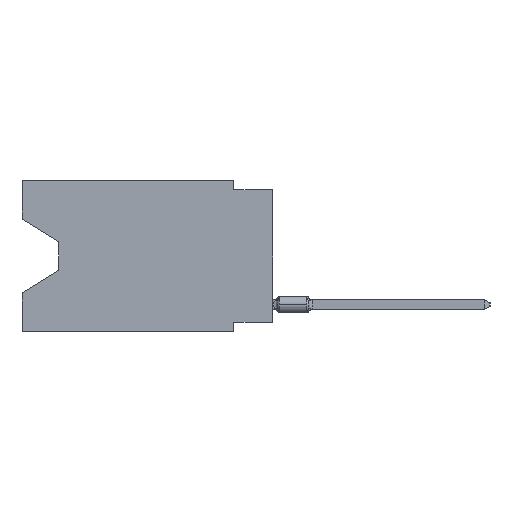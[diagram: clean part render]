
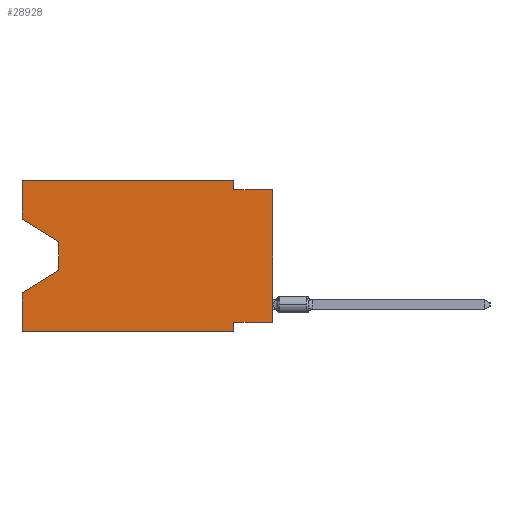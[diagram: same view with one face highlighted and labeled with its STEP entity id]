
A CAD part, left-side view. The second image highlights one B-rep face of the part: STEP entity #28928.
In plain terms, the highlighted planar face has unit normal (-1, 0, 0).
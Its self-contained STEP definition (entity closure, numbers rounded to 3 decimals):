
#574 = CARTESIAN_POINT ( 'NONE',  ( 0., 13.97, -4.013 ) ) ;
#907 = CARTESIAN_POINT ( 'NONE',  ( 0., 16.383, -7.36 ) ) ;
#1295 = DIRECTION ( 'NONE',  ( 0., -0.855, -0.519 ) ) ;
#1800 = VECTOR ( 'NONE', #1828, 1000. ) ;
#1828 = DIRECTION ( 'NONE',  ( 0., 1., 0. ) ) ;
#1912 = VECTOR ( 'NONE', #26800, 1000. ) ;
#1988 = AXIS2_PLACEMENT_3D ( 'NONE', #5019, #26627, #13633 ) ;
#2088 = EDGE_CURVE ( 'NONE', #6291, #32287, #13755, .T. ) ;
#2359 = CARTESIAN_POINT ( 'NONE',  ( 0., 16.383, -9.906 ) ) ;
#2468 = EDGE_CURVE ( 'NONE', #8703, #30453, #21940, .T. ) ;
#2623 = LINE ( 'NONE', #15472, #23914 ) ;
#2914 = CARTESIAN_POINT ( 'NONE',  ( 0., 16.383, -2.546 ) ) ;
#3420 = CARTESIAN_POINT ( 'NONE',  ( 0., 2.54, 0. ) ) ;
#3566 = ORIENTED_EDGE ( 'NONE', *, *, #20096, .T. ) ;
#3781 = DIRECTION ( 'NONE',  ( 0., 0.855, -0.519 ) ) ;
#3943 = CARTESIAN_POINT ( 'NONE',  ( 0., 2.54, -9.906 ) ) ;
#5019 = CARTESIAN_POINT ( 'NONE',  ( 0., 16.383, 0. ) ) ;
#5112 = DIRECTION ( 'NONE',  ( 0., 0., 1. ) ) ;
#5271 = DIRECTION ( 'NONE',  ( 0., -1., 0. ) ) ;
#6037 = DIRECTION ( 'NONE',  ( 0., 0., 1. ) ) ;
#6098 = VECTOR ( 'NONE', #5271, 1000. ) ;
#6171 = ORIENTED_EDGE ( 'NONE', *, *, #2088, .T. ) ;
#6291 = VERTEX_POINT ( 'NONE', #31107 ) ;
#7179 = CARTESIAN_POINT ( 'NONE',  ( 0., 0., -0.635 ) ) ;
#7238 = ORIENTED_EDGE ( 'NONE', *, *, #2468, .T. ) ;
#7277 = CARTESIAN_POINT ( 'NONE',  ( 0., 16.383, 0. ) ) ;
#7538 = VERTEX_POINT ( 'NONE', #18780 ) ;
#7618 = VECTOR ( 'NONE', #1295, 1000. ) ;
#8472 = DIRECTION ( 'NONE',  ( 0., 0., -1. ) ) ;
#8703 = VERTEX_POINT ( 'NONE', #2359 ) ;
#9199 = LINE ( 'NONE', #14657, #1800 ) ;
#9858 = EDGE_CURVE ( 'NONE', #22344, #11914, #17973, .T. ) ;
#10079 = CARTESIAN_POINT ( 'NONE',  ( 0., 2.54, 0. ) ) ;
#10644 = EDGE_CURVE ( 'NONE', #11914, #33582, #23516, .T. ) ;
#11840 = ORIENTED_EDGE ( 'NONE', *, *, #10644, .F. ) ;
#11914 = VERTEX_POINT ( 'NONE', #31390 ) ;
#13205 = VECTOR ( 'NONE', #23246, 1000. ) ;
#13214 = CARTESIAN_POINT ( 'NONE',  ( 0., 16.383, 0. ) ) ;
#13633 = DIRECTION ( 'NONE',  ( 0., 0., -1. ) ) ;
#13713 = ORIENTED_EDGE ( 'NONE', *, *, #30791, .T. ) ;
#13755 = LINE ( 'NONE', #574, #25171 ) ;
#14209 = VERTEX_POINT ( 'NONE', #7277 ) ;
#14579 = CARTESIAN_POINT ( 'NONE',  ( 0., 0., -0.635 ) ) ;
#14657 = CARTESIAN_POINT ( 'NONE',  ( 0., 0., -9.271 ) ) ;
#14918 = CARTESIAN_POINT ( 'NONE',  ( 0., 0., -9.271 ) ) ;
#14926 = ORIENTED_EDGE ( 'NONE', *, *, #25609, .F. ) ;
#15129 = EDGE_CURVE ( 'NONE', #23549, #14209, #19733, .T. ) ;
#15472 = CARTESIAN_POINT ( 'NONE',  ( 0., 0., 0. ) ) ;
#15497 = EDGE_CURVE ( 'NONE', #7538, #30453, #16725, .T. ) ;
#16527 = VECTOR ( 'NONE', #34241, 1000. ) ;
#16557 = DIRECTION ( 'NONE',  ( 0., 0., -1. ) ) ;
#16686 = CARTESIAN_POINT ( 'NONE',  ( 0., 16.383, -9.906 ) ) ;
#16725 = LINE ( 'NONE', #27610, #19671 ) ;
#17438 = VECTOR ( 'NONE', #6037, 1000. ) ;
#17606 = CARTESIAN_POINT ( 'NONE',  ( 0., 16.383, -2.546 ) ) ;
#17973 = LINE ( 'NONE', #10079, #13205 ) ;
#18780 = CARTESIAN_POINT ( 'NONE',  ( 0., 2.54, -9.271 ) ) ;
#18956 = EDGE_CURVE ( 'NONE', #8703, #24749, #31817, .T. ) ;
#19671 = VECTOR ( 'NONE', #16557, 1000. ) ;
#19733 = LINE ( 'NONE', #27477, #17438 ) ;
#19958 = EDGE_CURVE ( 'NONE', #14209, #22344, #21692, .T. ) ;
#20096 = EDGE_CURVE ( 'NONE', #32287, #24749, #25394, .T. ) ;
#21394 = CARTESIAN_POINT ( 'NONE',  ( 0., 13.97, -5.893 ) ) ;
#21692 = LINE ( 'NONE', #32421, #1912 ) ;
#21940 = LINE ( 'NONE', #16686, #6098 ) ;
#22344 = VERTEX_POINT ( 'NONE', #3420 ) ;
#23246 = DIRECTION ( 'NONE',  ( 0., 0., -1. ) ) ;
#23516 = LINE ( 'NONE', #7179, #16527 ) ;
#23549 = VERTEX_POINT ( 'NONE', #2914 ) ;
#23710 = VECTOR ( 'NONE', #5112, 1000. ) ;
#23914 = VECTOR ( 'NONE', #26342, 1000. ) ;
#23980 = FACE_OUTER_BOUND ( 'NONE', #30723, .T. ) ;
#24288 = VERTEX_POINT ( 'NONE', #14918 ) ;
#24749 = VERTEX_POINT ( 'NONE', #907 ) ;
#25171 = VECTOR ( 'NONE', #8472, 1000. ) ;
#25394 = LINE ( 'NONE', #30305, #26015 ) ;
#25609 = EDGE_CURVE ( 'NONE', #24288, #7538, #9199, .T. ) ;
#26015 = VECTOR ( 'NONE', #3781, 1000. ) ;
#26342 = DIRECTION ( 'NONE',  ( 0., 0., 1. ) ) ;
#26627 = DIRECTION ( 'NONE',  ( 1., 0., 0. ) ) ;
#26800 = DIRECTION ( 'NONE',  ( 0., -1., 0. ) ) ;
#26869 = ORIENTED_EDGE ( 'NONE', *, *, #15129, .F. ) ;
#26940 = ORIENTED_EDGE ( 'NONE', *, *, #19958, .F. ) ;
#27100 = ORIENTED_EDGE ( 'NONE', *, *, #31352, .T. ) ;
#27477 = CARTESIAN_POINT ( 'NONE',  ( 0., 16.383, 0. ) ) ;
#27610 = CARTESIAN_POINT ( 'NONE',  ( 0., 2.54, -9.906 ) ) ;
#28077 = ORIENTED_EDGE ( 'NONE', *, *, #15497, .F. ) ;
#28928 = ADVANCED_FACE ( 'NONE', ( #23980 ), #34372, .F. ) ;
#30305 = CARTESIAN_POINT ( 'NONE',  ( 0., 13.97, -5.893 ) ) ;
#30453 = VERTEX_POINT ( 'NONE', #3943 ) ;
#30723 = EDGE_LOOP ( 'NONE', ( #13713, #6171, #3566, #33524, #7238, #28077, #14926, #27100, #11840, #31132, #26940, #26869 ) ) ;
#30791 = EDGE_CURVE ( 'NONE', #23549, #6291, #33767, .T. ) ;
#31107 = CARTESIAN_POINT ( 'NONE',  ( 0., 13.97, -4.013 ) ) ;
#31132 = ORIENTED_EDGE ( 'NONE', *, *, #9858, .F. ) ;
#31352 = EDGE_CURVE ( 'NONE', #24288, #33582, #2623, .T. ) ;
#31390 = CARTESIAN_POINT ( 'NONE',  ( 0., 2.54, -0.635 ) ) ;
#31817 = LINE ( 'NONE', #13214, #23710 ) ;
#32287 = VERTEX_POINT ( 'NONE', #21394 ) ;
#32421 = CARTESIAN_POINT ( 'NONE',  ( 0., 16.383, 0. ) ) ;
#33524 = ORIENTED_EDGE ( 'NONE', *, *, #18956, .F. ) ;
#33582 = VERTEX_POINT ( 'NONE', #14579 ) ;
#33767 = LINE ( 'NONE', #17606, #7618 ) ;
#34241 = DIRECTION ( 'NONE',  ( 0., -1., 0. ) ) ;
#34372 = PLANE ( 'NONE',  #1988 ) ;
